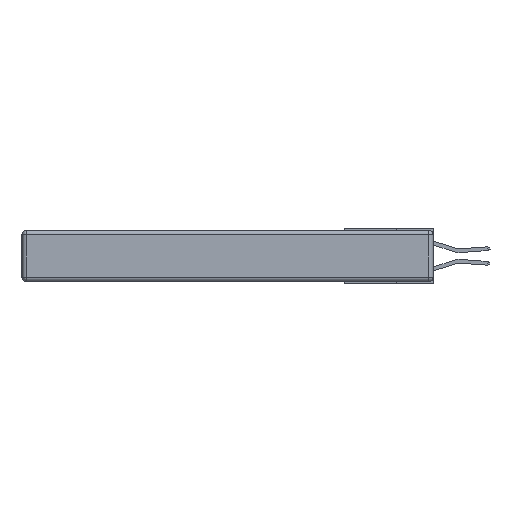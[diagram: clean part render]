
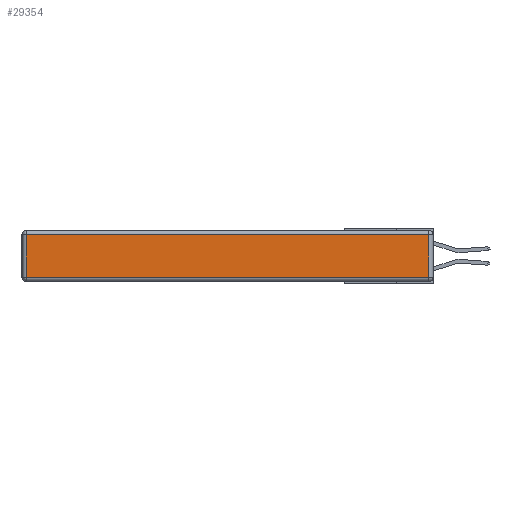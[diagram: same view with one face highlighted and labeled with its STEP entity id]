
A CAD part, left-side view. The second image highlights one B-rep face of the part: STEP entity #29354.
In plain terms, the highlighted planar face has unit normal (-1, 0, 0).
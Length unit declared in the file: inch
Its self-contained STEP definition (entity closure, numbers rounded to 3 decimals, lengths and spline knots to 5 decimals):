
#2076 = VECTOR ( 'NONE', #15589, 39.37008 ) ;
#2785 = VERTEX_POINT ( 'NONE', #12265 ) ;
#4837 = ORIENTED_EDGE ( 'NONE', *, *, #25668, .T. ) ;
#5937 = VERTEX_POINT ( 'NONE', #8270 ) ;
#8270 = CARTESIAN_POINT ( 'NONE',  ( 0., 0.03, -0.03 ) ) ;
#8661 = CARTESIAN_POINT ( 'NONE',  ( 0., 2.75, -0.03 ) ) ;
#9791 = EDGE_CURVE ( 'NONE', #5937, #29099, #25088, .T. ) ;
#10657 = LINE ( 'NONE', #15918, #27159 ) ;
#12265 = CARTESIAN_POINT ( 'NONE',  ( 0., 2.72, -0.313 ) ) ;
#15290 = CARTESIAN_POINT ( 'NONE',  ( 0., 0.03, -0.313 ) ) ;
#15325 = VERTEX_POINT ( 'NONE', #15290 ) ;
#15589 = DIRECTION ( 'NONE',  ( 0., -1., 0. ) ) ;
#15723 = EDGE_LOOP ( 'NONE', ( #19365, #4837, #25268, #21554 ) ) ;
#15918 = CARTESIAN_POINT ( 'NONE',  ( 0., 2.72, -0.343 ) ) ;
#15955 = EDGE_CURVE ( 'NONE', #2785, #15325, #28021, .T. ) ;
#16717 = CARTESIAN_POINT ( 'NONE',  ( 0., 2.72, -0.03 ) ) ;
#16828 = FACE_OUTER_BOUND ( 'NONE', #15723, .T. ) ;
#17427 = VECTOR ( 'NONE', #20500, 39.37008 ) ;
#17995 = CARTESIAN_POINT ( 'NONE',  ( 0., 0., -0.313 ) ) ;
#18336 = CARTESIAN_POINT ( 'NONE',  ( 0., 0., -0.343 ) ) ;
#19365 = ORIENTED_EDGE ( 'NONE', *, *, #15955, .T. ) ;
#20500 = DIRECTION ( 'NONE',  ( 0., 0., 1. ) ) ;
#21077 = PLANE ( 'NONE',  #30491 ) ;
#21097 = LINE ( 'NONE', #25581, #17427 ) ;
#21554 = ORIENTED_EDGE ( 'NONE', *, *, #26974, .T. ) ;
#22197 = DIRECTION ( 'NONE',  ( 0., 0., -1. ) ) ;
#23616 = DIRECTION ( 'NONE',  ( -1., 0., 0. ) ) ;
#23867 = VECTOR ( 'NONE', #24709, 39.37008 ) ;
#24709 = DIRECTION ( 'NONE',  ( 0., 1., 0. ) ) ;
#25088 = LINE ( 'NONE', #8661, #23867 ) ;
#25268 = ORIENTED_EDGE ( 'NONE', *, *, #9791, .T. ) ;
#25581 = CARTESIAN_POINT ( 'NONE',  ( 0., 0.03, -0.343 ) ) ;
#25668 = EDGE_CURVE ( 'NONE', #15325, #5937, #21097, .T. ) ;
#26132 = DIRECTION ( 'NONE',  ( 0., 0., 1. ) ) ;
#26974 = EDGE_CURVE ( 'NONE', #29099, #2785, #10657, .T. ) ;
#27159 = VECTOR ( 'NONE', #22197, 39.37008 ) ;
#28021 = LINE ( 'NONE', #17995, #2076 ) ;
#29099 = VERTEX_POINT ( 'NONE', #16717 ) ;
#29354 = ADVANCED_FACE ( 'NONE', ( #16828 ), #21077, .T. ) ;
#30491 = AXIS2_PLACEMENT_3D ( 'NONE', #18336, #23616, #26132 ) ;
